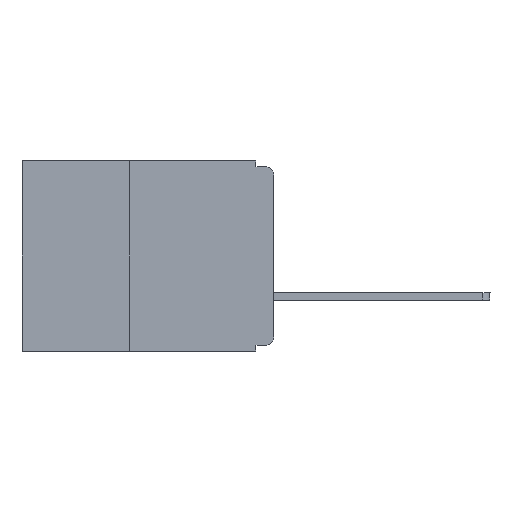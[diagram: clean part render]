
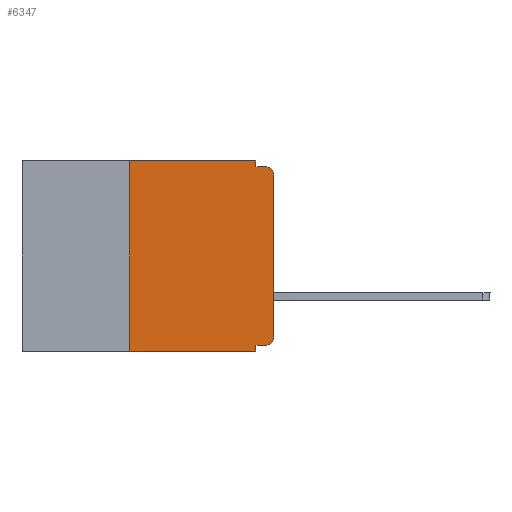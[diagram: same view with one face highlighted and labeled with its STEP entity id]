
A CAD part, left-side view. The second image highlights one B-rep face of the part: STEP entity #6347.
In plain terms, the highlighted planar face has unit normal (-1, 0, 0).
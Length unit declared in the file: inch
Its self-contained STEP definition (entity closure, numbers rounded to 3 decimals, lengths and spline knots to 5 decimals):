
#95 = AXIS2_PLACEMENT_3D ( 'NONE', #8890, #6932, #4929 ) ;
#257 = CARTESIAN_POINT ( 'NONE',  ( 0., 0.031, 0. ) ) ;
#494 = CARTESIAN_POINT ( 'NONE',  ( 0., 0.015, -0.32 ) ) ;
#519 = DIRECTION ( 'NONE',  ( 0., -1., 0. ) ) ;
#759 = CARTESIAN_POINT ( 'NONE',  ( 0., 0.015, -0.01 ) ) ;
#780 = CARTESIAN_POINT ( 'NONE',  ( 0., 0., -0.32 ) ) ;
#838 = CARTESIAN_POINT ( 'NONE',  ( 0., 0.031, -0.33 ) ) ;
#917 = EDGE_CURVE ( 'NONE', #5386, #3593, #3551, .T. ) ;
#1888 = EDGE_CURVE ( 'NONE', #9359, #9543, #5454, .T. ) ;
#1956 = ORIENTED_EDGE ( 'NONE', *, *, #2950, .F. ) ;
#2585 = DIRECTION ( 'NONE',  ( -1., 0., 0. ) ) ;
#2647 = VERTEX_POINT ( 'NONE', #5740 ) ;
#2748 = VECTOR ( 'NONE', #4906, 39.37008 ) ;
#2776 = CARTESIAN_POINT ( 'NONE',  ( 0., 0., -0.305 ) ) ;
#2857 = CARTESIAN_POINT ( 'NONE',  ( 0., 0.031, -0.33 ) ) ;
#2950 = EDGE_CURVE ( 'NONE', #3576, #2647, #7315, .T. ) ;
#3087 = EDGE_CURVE ( 'NONE', #9359, #6313, #8243, .T. ) ;
#3210 = ORIENTED_EDGE ( 'NONE', *, *, #9257, .F. ) ;
#3543 = CARTESIAN_POINT ( 'NONE',  ( 0., 0., 0. ) ) ;
#3551 = LINE ( 'NONE', #780, #11956 ) ;
#3563 = CARTESIAN_POINT ( 'NONE',  ( 0., 0.015, -0.305 ) ) ;
#3576 = VERTEX_POINT ( 'NONE', #7844 ) ;
#3593 = VERTEX_POINT ( 'NONE', #6112 ) ;
#3693 = CIRCLE ( 'NONE', #4166, 0.015 ) ;
#3753 = VECTOR ( 'NONE', #12263, 39.37008 ) ;
#3766 = ORIENTED_EDGE ( 'NONE', *, *, #1888, .F. ) ;
#3812 = ORIENTED_EDGE ( 'NONE', *, *, #5388, .F. ) ;
#3848 = EDGE_CURVE ( 'NONE', #6434, #8143, #3693, .T. ) ;
#4107 = VECTOR ( 'NONE', #10369, 39.37008 ) ;
#4152 = CIRCLE ( 'NONE', #6530, 0.015 ) ;
#4166 = AXIS2_PLACEMENT_3D ( 'NONE', #6639, #4560, #8670 ) ;
#4560 = DIRECTION ( 'NONE',  ( -1., 0., 0. ) ) ;
#4791 = CARTESIAN_POINT ( 'NONE',  ( 0., 0., -0.025 ) ) ;
#4906 = DIRECTION ( 'NONE',  ( 0., -1., 0. ) ) ;
#4929 = DIRECTION ( 'NONE',  ( 0., 0., -1. ) ) ;
#5386 = VERTEX_POINT ( 'NONE', #494 ) ;
#5388 = EDGE_CURVE ( 'NONE', #9543, #3576, #9373, .T. ) ;
#5451 = CARTESIAN_POINT ( 'NONE',  ( 0., 0.25, 0. ) ) ;
#5454 = LINE ( 'NONE', #10226, #3753 ) ;
#5558 = EDGE_CURVE ( 'NONE', #3593, #6313, #6244, .T. ) ;
#5564 = VECTOR ( 'NONE', #519, 39.37008 ) ;
#5740 = CARTESIAN_POINT ( 'NONE',  ( 0., 0.031, -0.01 ) ) ;
#5866 = ORIENTED_EDGE ( 'NONE', *, *, #3848, .T. ) ;
#6098 = VECTOR ( 'NONE', #9365, 39.37008 ) ;
#6112 = CARTESIAN_POINT ( 'NONE',  ( 0., 0.031, -0.32 ) ) ;
#6244 = LINE ( 'NONE', #2857, #9966 ) ;
#6313 = VERTEX_POINT ( 'NONE', #838 ) ;
#6347 = ADVANCED_FACE ( 'NONE', ( #8100 ), #12861, .F. ) ;
#6434 = VERTEX_POINT ( 'NONE', #4791 ) ;
#6442 = CARTESIAN_POINT ( 'NONE',  ( 0., 0.437, 0. ) ) ;
#6530 = AXIS2_PLACEMENT_3D ( 'NONE', #3563, #2585, #10522 ) ;
#6639 = CARTESIAN_POINT ( 'NONE',  ( 0., 0.015, -0.025 ) ) ;
#6932 = DIRECTION ( 'NONE',  ( 1., 0., 0. ) ) ;
#7315 = LINE ( 'NONE', #257, #8567 ) ;
#7738 = ORIENTED_EDGE ( 'NONE', *, *, #12222, .T. ) ;
#7844 = CARTESIAN_POINT ( 'NONE',  ( 0., 0.031, 0. ) ) ;
#7893 = ORIENTED_EDGE ( 'NONE', *, *, #8586, .T. ) ;
#8082 = VERTEX_POINT ( 'NONE', #2776 ) ;
#8100 = FACE_OUTER_BOUND ( 'NONE', #8326, .T. ) ;
#8143 = VERTEX_POINT ( 'NONE', #759 ) ;
#8160 = LINE ( 'NONE', #3543, #4107 ) ;
#8243 = LINE ( 'NONE', #10422, #5564 ) ;
#8326 = EDGE_LOOP ( 'NONE', ( #7738, #5866, #3210, #1956, #3812, #3766, #11954, #9950, #10286, #7893 ) ) ;
#8567 = VECTOR ( 'NONE', #10380, 39.37008 ) ;
#8586 = EDGE_CURVE ( 'NONE', #5386, #8082, #4152, .T. ) ;
#8670 = DIRECTION ( 'NONE',  ( 0., 0., -1. ) ) ;
#8890 = CARTESIAN_POINT ( 'NONE',  ( 0., 0.437, 0. ) ) ;
#8998 = CARTESIAN_POINT ( 'NONE',  ( 0., 0., -0.01 ) ) ;
#9072 = CARTESIAN_POINT ( 'NONE',  ( 0., 0.25, -0.33 ) ) ;
#9257 = EDGE_CURVE ( 'NONE', #2647, #8143, #10021, .T. ) ;
#9359 = VERTEX_POINT ( 'NONE', #9072 ) ;
#9365 = DIRECTION ( 'NONE',  ( 0., -1., 0. ) ) ;
#9373 = LINE ( 'NONE', #6442, #6098 ) ;
#9543 = VERTEX_POINT ( 'NONE', #5451 ) ;
#9868 = DIRECTION ( 'NONE',  ( 0., 0., -1. ) ) ;
#9950 = ORIENTED_EDGE ( 'NONE', *, *, #5558, .F. ) ;
#9966 = VECTOR ( 'NONE', #9868, 39.37008 ) ;
#10021 = LINE ( 'NONE', #8998, #2748 ) ;
#10226 = CARTESIAN_POINT ( 'NONE',  ( 0., 0.25, -0.33 ) ) ;
#10286 = ORIENTED_EDGE ( 'NONE', *, *, #917, .F. ) ;
#10369 = DIRECTION ( 'NONE',  ( 0., 0., 1. ) ) ;
#10380 = DIRECTION ( 'NONE',  ( 0., 0., -1. ) ) ;
#10422 = CARTESIAN_POINT ( 'NONE',  ( 0., 0.437, -0.33 ) ) ;
#10522 = DIRECTION ( 'NONE',  ( 0., 0., -1. ) ) ;
#11954 = ORIENTED_EDGE ( 'NONE', *, *, #3087, .T. ) ;
#11956 = VECTOR ( 'NONE', #12739, 39.37008 ) ;
#12222 = EDGE_CURVE ( 'NONE', #8082, #6434, #8160, .T. ) ;
#12263 = DIRECTION ( 'NONE',  ( 0., 0., 1. ) ) ;
#12739 = DIRECTION ( 'NONE',  ( 0., 1., 0. ) ) ;
#12861 = PLANE ( 'NONE',  #95 ) ;
